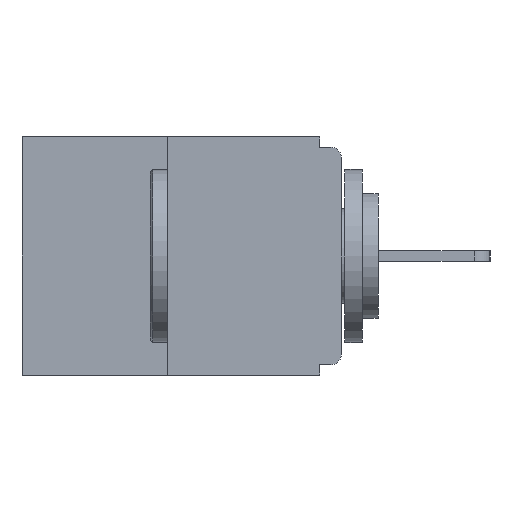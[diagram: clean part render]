
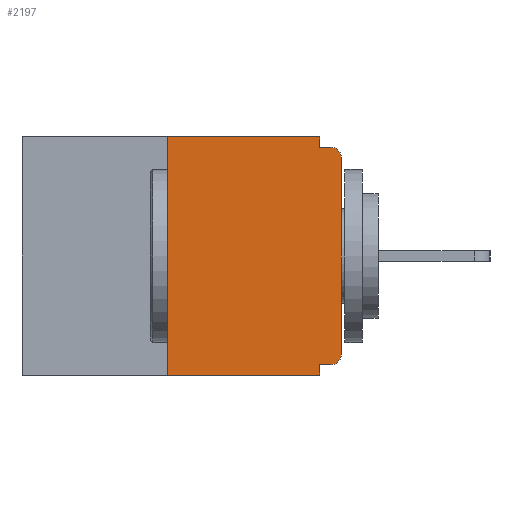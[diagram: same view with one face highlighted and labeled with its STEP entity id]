
A CAD part, left-side view. The second image highlights one B-rep face of the part: STEP entity #2197.
In plain terms, the highlighted planar face has unit normal (-1, 0, 0).
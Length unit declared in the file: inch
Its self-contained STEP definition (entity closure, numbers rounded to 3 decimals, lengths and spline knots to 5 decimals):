
#46 = CARTESIAN_POINT ( 'NONE',  ( 0., 0.015, -0.015 ) ) ;
#380 = EDGE_CURVE ( 'NONE', #12304, #745, #13228, .T. ) ;
#436 = VECTOR ( 'NONE', #11248, 39.37008 ) ;
#520 = EDGE_CURVE ( 'NONE', #598, #5227, #11914, .T. ) ;
#598 = VERTEX_POINT ( 'NONE', #14406 ) ;
#687 = CARTESIAN_POINT ( 'NONE',  ( 0., 0.25, -0.343 ) ) ;
#734 = VECTOR ( 'NONE', #10849, 39.37008 ) ;
#745 = VERTEX_POINT ( 'NONE', #3811 ) ;
#787 = ORIENTED_EDGE ( 'NONE', *, *, #4458, .F. ) ;
#1022 = DIRECTION ( 'NONE',  ( 0., 0., 1. ) ) ;
#1124 = CARTESIAN_POINT ( 'NONE',  ( 0., 0.46, 0. ) ) ;
#1127 = VERTEX_POINT ( 'NONE', #687 ) ;
#1345 = CARTESIAN_POINT ( 'NONE',  ( 0., 0.031, -0.343 ) ) ;
#1402 = VERTEX_POINT ( 'NONE', #14264 ) ;
#1929 = CARTESIAN_POINT ( 'NONE',  ( 0., 0.031, -0.015 ) ) ;
#2154 = AXIS2_PLACEMENT_3D ( 'NONE', #3995, #4015, #6029 ) ;
#2171 = CARTESIAN_POINT ( 'NONE',  ( 0., 0.25, 0. ) ) ;
#2197 = ADVANCED_FACE ( 'NONE', ( #2374 ), #10000, .F. ) ;
#2309 = DIRECTION ( 'NONE',  ( 0., 0., 1. ) ) ;
#2374 = FACE_OUTER_BOUND ( 'NONE', #9788, .T. ) ;
#2464 = CARTESIAN_POINT ( 'NONE',  ( 0., 0.25, 0. ) ) ;
#2812 = EDGE_CURVE ( 'NONE', #4153, #9866, #6788, .T. ) ;
#2921 = CARTESIAN_POINT ( 'NONE',  ( 0., 0.031, 0. ) ) ;
#2997 = VECTOR ( 'NONE', #1022, 39.37008 ) ;
#3167 = DIRECTION ( 'NONE',  ( 0., 1., 0. ) ) ;
#3357 = EDGE_CURVE ( 'NONE', #5227, #4886, #8699, .T. ) ;
#3515 = LINE ( 'NONE', #2921, #734 ) ;
#3548 = EDGE_CURVE ( 'NONE', #1127, #4886, #14421, .T. ) ;
#3811 = CARTESIAN_POINT ( 'NONE',  ( 0., 0.031, 0. ) ) ;
#3995 = CARTESIAN_POINT ( 'NONE',  ( 0., 0.015, -0.03 ) ) ;
#4015 = DIRECTION ( 'NONE',  ( -1., 0., 0. ) ) ;
#4153 = VERTEX_POINT ( 'NONE', #1929 ) ;
#4311 = ORIENTED_EDGE ( 'NONE', *, *, #520, .F. ) ;
#4458 = EDGE_CURVE ( 'NONE', #1127, #12304, #6542, .T. ) ;
#4466 = DIRECTION ( 'NONE',  ( -1., 0., 0. ) ) ;
#4692 = ORIENTED_EDGE ( 'NONE', *, *, #10298, .T. ) ;
#4886 = VERTEX_POINT ( 'NONE', #11373 ) ;
#5049 = ORIENTED_EDGE ( 'NONE', *, *, #11917, .F. ) ;
#5227 = VERTEX_POINT ( 'NONE', #8012 ) ;
#5633 = VECTOR ( 'NONE', #6288, 39.37008 ) ;
#5802 = CARTESIAN_POINT ( 'NONE',  ( 0., 0., 0. ) ) ;
#6029 = DIRECTION ( 'NONE',  ( 0., 0., -1. ) ) ;
#6285 = DIRECTION ( 'NONE',  ( 0., 0., -1. ) ) ;
#6288 = DIRECTION ( 'NONE',  ( 0., 0., -1. ) ) ;
#6345 = AXIS2_PLACEMENT_3D ( 'NONE', #9998, #10176, #6285 ) ;
#6542 = LINE ( 'NONE', #2171, #2997 ) ;
#6788 = LINE ( 'NONE', #11362, #436 ) ;
#7089 = ORIENTED_EDGE ( 'NONE', *, *, #3548, .T. ) ;
#7771 = ORIENTED_EDGE ( 'NONE', *, *, #7858, .T. ) ;
#7858 = EDGE_CURVE ( 'NONE', #1402, #9866, #8927, .T. ) ;
#8012 = CARTESIAN_POINT ( 'NONE',  ( 0., 0.031, -0.328 ) ) ;
#8256 = CARTESIAN_POINT ( 'NONE',  ( 0., 0., -0.313 ) ) ;
#8699 = LINE ( 'NONE', #1345, #5633 ) ;
#8927 = CIRCLE ( 'NONE', #2154, 0.015 ) ;
#9010 = DIRECTION ( 'NONE',  ( 0., -1., 0. ) ) ;
#9101 = VECTOR ( 'NONE', #3167, 39.37008 ) ;
#9671 = ORIENTED_EDGE ( 'NONE', *, *, #380, .F. ) ;
#9781 = DIRECTION ( 'NONE',  ( 0., -1., 0. ) ) ;
#9788 = EDGE_LOOP ( 'NONE', ( #9671, #787, #7089, #9990, #4311, #10335, #4692, #7771, #13480, #5049 ) ) ;
#9866 = VERTEX_POINT ( 'NONE', #46 ) ;
#9990 = ORIENTED_EDGE ( 'NONE', *, *, #3357, .F. ) ;
#9998 = CARTESIAN_POINT ( 'NONE',  ( 0., 0.46, 0. ) ) ;
#10000 = PLANE ( 'NONE',  #6345 ) ;
#10176 = DIRECTION ( 'NONE',  ( 1., 0., 0. ) ) ;
#10298 = EDGE_CURVE ( 'NONE', #10363, #1402, #13343, .T. ) ;
#10335 = ORIENTED_EDGE ( 'NONE', *, *, #14202, .T. ) ;
#10363 = VERTEX_POINT ( 'NONE', #8256 ) ;
#10428 = VECTOR ( 'NONE', #9010, 39.37008 ) ;
#10538 = VECTOR ( 'NONE', #2309, 39.37008 ) ;
#10849 = DIRECTION ( 'NONE',  ( 0., 0., -1. ) ) ;
#10967 = CARTESIAN_POINT ( 'NONE',  ( 0., 0., -0.328 ) ) ;
#11055 = CARTESIAN_POINT ( 'NONE',  ( 0., 0.46, -0.343 ) ) ;
#11178 = CARTESIAN_POINT ( 'NONE',  ( 0., 0.015, -0.313 ) ) ;
#11248 = DIRECTION ( 'NONE',  ( 0., -1., 0. ) ) ;
#11362 = CARTESIAN_POINT ( 'NONE',  ( 0., 0., -0.015 ) ) ;
#11373 = CARTESIAN_POINT ( 'NONE',  ( 0., 0.031, -0.343 ) ) ;
#11670 = VECTOR ( 'NONE', #9781, 39.37008 ) ;
#11914 = LINE ( 'NONE', #10967, #9101 ) ;
#11917 = EDGE_CURVE ( 'NONE', #745, #4153, #3515, .T. ) ;
#12245 = DIRECTION ( 'NONE',  ( 0., 0., -1. ) ) ;
#12304 = VERTEX_POINT ( 'NONE', #2464 ) ;
#13188 = CIRCLE ( 'NONE', #14016, 0.015 ) ;
#13228 = LINE ( 'NONE', #1124, #10428 ) ;
#13343 = LINE ( 'NONE', #5802, #10538 ) ;
#13480 = ORIENTED_EDGE ( 'NONE', *, *, #2812, .F. ) ;
#14016 = AXIS2_PLACEMENT_3D ( 'NONE', #11178, #4466, #12245 ) ;
#14202 = EDGE_CURVE ( 'NONE', #598, #10363, #13188, .T. ) ;
#14264 = CARTESIAN_POINT ( 'NONE',  ( 0., 0., -0.03 ) ) ;
#14406 = CARTESIAN_POINT ( 'NONE',  ( 0., 0.015, -0.328 ) ) ;
#14421 = LINE ( 'NONE', #11055, #11670 ) ;
